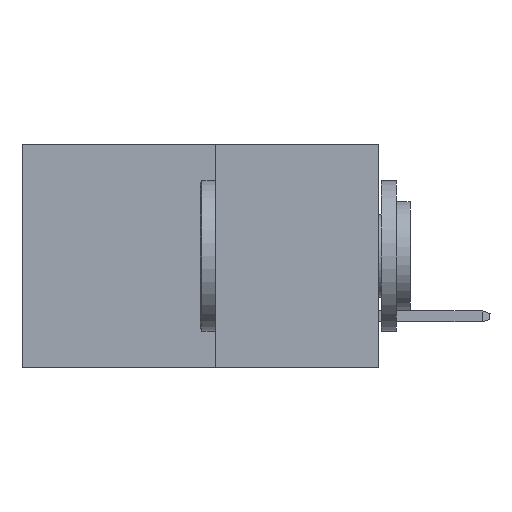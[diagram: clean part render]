
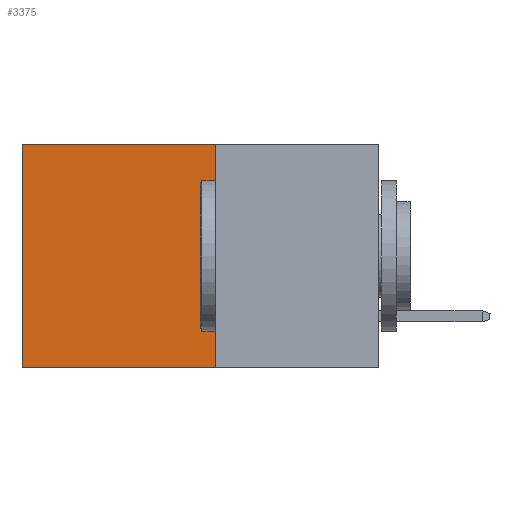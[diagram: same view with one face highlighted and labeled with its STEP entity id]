
A CAD part, left-side view. The second image highlights one B-rep face of the part: STEP entity #3375.
In plain terms, the highlighted planar face has unit normal (-1, 0, 0).
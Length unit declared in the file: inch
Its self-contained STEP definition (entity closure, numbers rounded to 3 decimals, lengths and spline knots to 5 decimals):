
#82 = DIRECTION ( 'NONE',  ( 0., 0., -1. ) ) ;
#207 = LINE ( 'NONE', #13160, #9986 ) ;
#211 = LINE ( 'NONE', #10291, #9044 ) ;
#1820 = EDGE_CURVE ( 'NONE', #14014, #3556, #14087, .T. ) ;
#2791 = ORIENTED_EDGE ( 'NONE', *, *, #1820, .F. ) ;
#2880 = EDGE_CURVE ( 'NONE', #10069, #14014, #12831, .T. ) ;
#3375 = ADVANCED_FACE ( 'NONE', ( #11223 ), #12955, .F. ) ;
#3544 = ORIENTED_EDGE ( 'NONE', *, *, #2880, .F. ) ;
#3556 = VERTEX_POINT ( 'NONE', #7746 ) ;
#3578 = CARTESIAN_POINT ( 'NONE',  ( 0.277, 0.27, -0.37 ) ) ;
#4244 = EDGE_LOOP ( 'NONE', ( #12997, #2791, #3544, #6486 ) ) ;
#5972 = CARTESIAN_POINT ( 'NONE',  ( 0.277, 0.27, 0. ) ) ;
#6486 = ORIENTED_EDGE ( 'NONE', *, *, #6837, .T. ) ;
#6837 = EDGE_CURVE ( 'NONE', #10069, #13858, #207, .T. ) ;
#7072 = DIRECTION ( 'NONE',  ( 0., 1., 0. ) ) ;
#7399 = VECTOR ( 'NONE', #8930, 39.37008 ) ;
#7746 = CARTESIAN_POINT ( 'NONE',  ( 0.277, 0.59, -0.37 ) ) ;
#7823 = EDGE_CURVE ( 'NONE', #13858, #3556, #211, .T. ) ;
#8666 = AXIS2_PLACEMENT_3D ( 'NONE', #12692, #12666, #12628 ) ;
#8930 = DIRECTION ( 'NONE',  ( 0., 0., -1. ) ) ;
#8984 = CARTESIAN_POINT ( 'NONE',  ( 0.277, 0.27, -0.37 ) ) ;
#9044 = VECTOR ( 'NONE', #82, 39.37008 ) ;
#9986 = VECTOR ( 'NONE', #7072, 39.37008 ) ;
#10069 = VERTEX_POINT ( 'NONE', #5972 ) ;
#10291 = CARTESIAN_POINT ( 'NONE',  ( 0.277, 0.59, -0.37 ) ) ;
#10585 = DIRECTION ( 'NONE',  ( 0., 1., 0. ) ) ;
#11223 = FACE_OUTER_BOUND ( 'NONE', #4244, .T. ) ;
#11511 = VECTOR ( 'NONE', #10585, 39.37008 ) ;
#11639 = CARTESIAN_POINT ( 'NONE',  ( 0.277, 0.59, 0. ) ) ;
#12628 = DIRECTION ( 'NONE',  ( 0., 0., -1. ) ) ;
#12666 = DIRECTION ( 'NONE',  ( 1., 0., 0. ) ) ;
#12692 = CARTESIAN_POINT ( 'NONE',  ( 0.277, 0.27, -0.37 ) ) ;
#12747 = CARTESIAN_POINT ( 'NONE',  ( 0.277, 0.27, -0.37 ) ) ;
#12831 = LINE ( 'NONE', #8984, #7399 ) ;
#12955 = PLANE ( 'NONE',  #8666 ) ;
#12997 = ORIENTED_EDGE ( 'NONE', *, *, #7823, .T. ) ;
#13160 = CARTESIAN_POINT ( 'NONE',  ( 0.277, 0.27, 0. ) ) ;
#13858 = VERTEX_POINT ( 'NONE', #11639 ) ;
#14014 = VERTEX_POINT ( 'NONE', #12747 ) ;
#14087 = LINE ( 'NONE', #3578, #11511 ) ;
